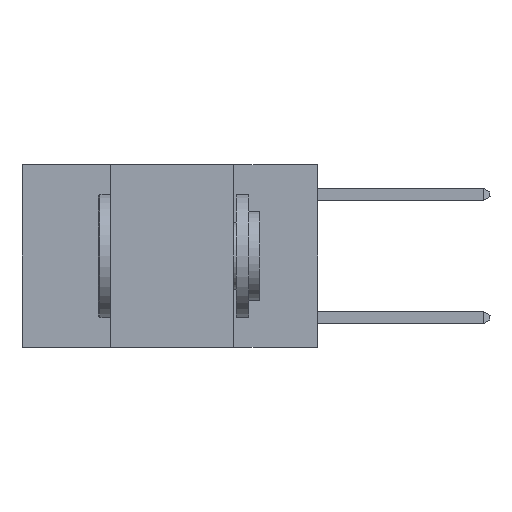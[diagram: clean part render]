
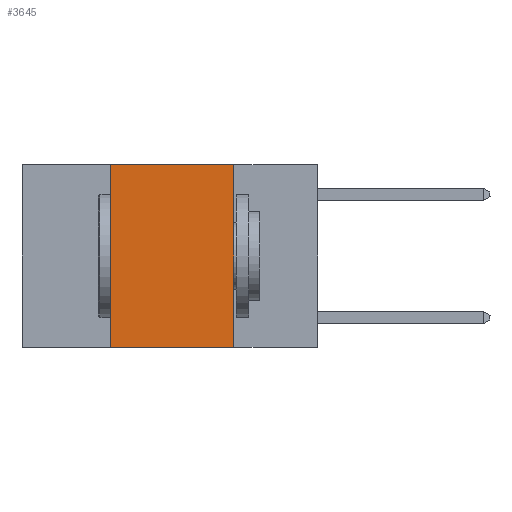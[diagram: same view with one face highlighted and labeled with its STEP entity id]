
A CAD part, left-side view. The second image highlights one B-rep face of the part: STEP entity #3645.
In plain terms, the highlighted planar face has unit normal (-1, 0, 0).
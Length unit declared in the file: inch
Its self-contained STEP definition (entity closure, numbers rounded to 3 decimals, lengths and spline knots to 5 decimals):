
#592 = CARTESIAN_POINT ( 'NONE',  ( 0., 0.17, 0. ) ) ;
#1279 = DIRECTION ( 'NONE',  ( 0., 0., 1. ) ) ;
#1818 = VERTEX_POINT ( 'NONE', #3105 ) ;
#2459 = VECTOR ( 'NONE', #17810, 39.37008 ) ;
#2551 = EDGE_CURVE ( 'NONE', #27510, #1818, #11614, .T. ) ;
#2915 = DIRECTION ( 'NONE',  ( 1., 0., 0. ) ) ;
#3105 = CARTESIAN_POINT ( 'NONE',  ( 0., 0.17, -0.37 ) ) ;
#3441 = ORIENTED_EDGE ( 'NONE', *, *, #21759, .F. ) ;
#3506 = CARTESIAN_POINT ( 'NONE',  ( 0., 0.17, 0. ) ) ;
#3531 = PLANE ( 'NONE',  #10000 ) ;
#3645 = ADVANCED_FACE ( 'NONE', ( #29089 ), #3531, .F. ) ;
#4856 = EDGE_LOOP ( 'NONE', ( #10980, #11847, #3441, #22394 ) ) ;
#5992 = VECTOR ( 'NONE', #1279, 39.37008 ) ;
#7222 = EDGE_CURVE ( 'NONE', #10058, #1818, #8347, .T. ) ;
#7468 = EDGE_CURVE ( 'NONE', #21597, #10058, #14532, .T. ) ;
#8347 = LINE ( 'NONE', #3506, #2459 ) ;
#9584 = CARTESIAN_POINT ( 'NONE',  ( 0., 0.6, 0. ) ) ;
#9606 = DIRECTION ( 'NONE',  ( 0., -1., 0. ) ) ;
#9664 = CARTESIAN_POINT ( 'NONE',  ( 0., 0.42, -0.37 ) ) ;
#10000 = AXIS2_PLACEMENT_3D ( 'NONE', #27059, #2915, #14894 ) ;
#10058 = VERTEX_POINT ( 'NONE', #592 ) ;
#10916 = VECTOR ( 'NONE', #26688, 39.37008 ) ;
#10980 = ORIENTED_EDGE ( 'NONE', *, *, #7222, .F. ) ;
#11614 = LINE ( 'NONE', #21258, #12218 ) ;
#11847 = ORIENTED_EDGE ( 'NONE', *, *, #7468, .F. ) ;
#12218 = VECTOR ( 'NONE', #9606, 39.37008 ) ;
#14532 = LINE ( 'NONE', #9584, #10916 ) ;
#14894 = DIRECTION ( 'NONE',  ( 0., 0., -1. ) ) ;
#15744 = CARTESIAN_POINT ( 'NONE',  ( 0., 0.42, 0. ) ) ;
#15899 = LINE ( 'NONE', #15744, #5992 ) ;
#17303 = CARTESIAN_POINT ( 'NONE',  ( 0., 0.42, 0. ) ) ;
#17810 = DIRECTION ( 'NONE',  ( 0., 0., -1. ) ) ;
#21258 = CARTESIAN_POINT ( 'NONE',  ( 0., 0.6, -0.37 ) ) ;
#21597 = VERTEX_POINT ( 'NONE', #17303 ) ;
#21759 = EDGE_CURVE ( 'NONE', #27510, #21597, #15899, .T. ) ;
#22394 = ORIENTED_EDGE ( 'NONE', *, *, #2551, .T. ) ;
#26688 = DIRECTION ( 'NONE',  ( 0., -1., 0. ) ) ;
#27059 = CARTESIAN_POINT ( 'NONE',  ( 0., 0.6, 0. ) ) ;
#27510 = VERTEX_POINT ( 'NONE', #9664 ) ;
#29089 = FACE_OUTER_BOUND ( 'NONE', #4856, .T. ) ;
